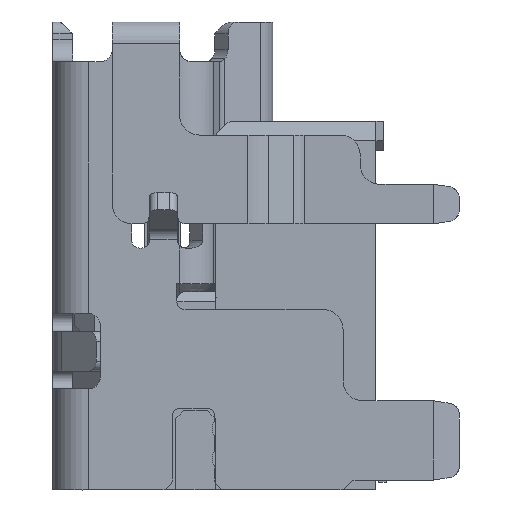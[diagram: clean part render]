
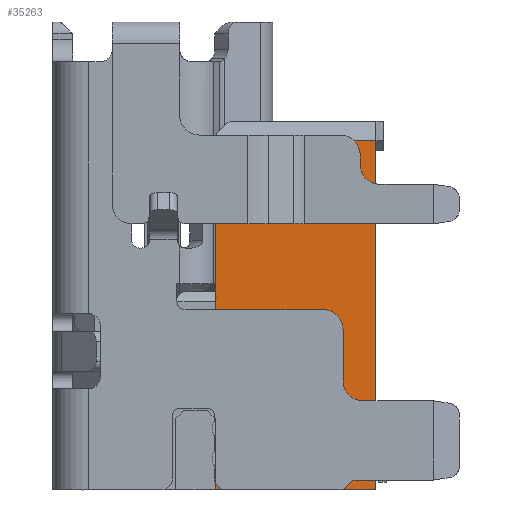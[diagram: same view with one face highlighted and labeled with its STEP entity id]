
A CAD part, left-side view. The second image highlights one B-rep face of the part: STEP entity #35263.
In plain terms, the highlighted planar face has unit normal (-1, 0, 0).
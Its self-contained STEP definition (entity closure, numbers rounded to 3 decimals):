
#2791 = CARTESIAN_POINT ( 'NONE',  ( -6.95, -3.575, -4.9 ) ) ;
#2960 = EDGE_LOOP ( 'NONE', ( #64803, #53405, #57798, #7119, #57390 ) ) ;
#3508 = LINE ( 'NONE', #2791, #50852 ) ;
#7119 = ORIENTED_EDGE ( 'NONE', *, *, #30680, .T. ) ;
#8371 = EDGE_CURVE ( 'NONE', #31630, #37756, #25866, .T. ) ;
#15078 = CARTESIAN_POINT ( 'NONE',  ( -6.95, -7.625, -4.65 ) ) ;
#21367 = DIRECTION ( 'NONE',  ( 0., 0., -1. ) ) ;
#25866 = LINE ( 'NONE', #26198, #50155 ) ;
#26198 = CARTESIAN_POINT ( 'NONE',  ( -6.95, -5.6, -9.3 ) ) ;
#26658 = LINE ( 'NONE', #15078, #41161 ) ;
#30680 = EDGE_CURVE ( 'NONE', #51789, #47878, #3508, .T. ) ;
#31224 = CARTESIAN_POINT ( 'NONE',  ( -6.95, -3.575, -0.5 ) ) ;
#31630 = VERTEX_POINT ( 'NONE', #64844 ) ;
#31987 = DIRECTION ( 'NONE',  ( 0., -1., 0. ) ) ;
#34311 = CARTESIAN_POINT ( 'NONE',  ( -6.95, -3.494, -9.476 ) ) ;
#34691 = DIRECTION ( 'NONE',  ( 0., -1., 0. ) ) ;
#35075 = DIRECTION ( 'NONE',  ( 0., 0., -1. ) ) ;
#35263 = ADVANCED_FACE ( 'NONE', ( #49933 ), #57509, .T. ) ;
#35579 = CARTESIAN_POINT ( 'NONE',  ( -6.95, -3.575, -4.5 ) ) ;
#37756 = VERTEX_POINT ( 'NONE', #63409 ) ;
#39363 = CARTESIAN_POINT ( 'NONE',  ( -6.95, -7.625, -0.5 ) ) ;
#41161 = VECTOR ( 'NONE', #65431, 1000. ) ;
#43654 = EDGE_CURVE ( 'NONE', #47878, #31630, #64897, .T. ) ;
#45292 = EDGE_CURVE ( 'NONE', #52387, #51789, #66682, .T. ) ;
#47878 = VERTEX_POINT ( 'NONE', #35579 ) ;
#49933 = FACE_OUTER_BOUND ( 'NONE', #2960, .T. ) ;
#50155 = VECTOR ( 'NONE', #31987, 1000. ) ;
#50852 = VECTOR ( 'NONE', #35075, 1000. ) ;
#50974 = EDGE_CURVE ( 'NONE', #37756, #52387, #26658, .T. ) ;
#51789 = VERTEX_POINT ( 'NONE', #31224 ) ;
#52387 = VERTEX_POINT ( 'NONE', #39363 ) ;
#53405 = ORIENTED_EDGE ( 'NONE', *, *, #50974, .T. ) ;
#53669 = CARTESIAN_POINT ( 'NONE',  ( -6.95, -3.575, -4.9 ) ) ;
#56450 = DIRECTION ( 'NONE',  ( -1., 0., 0. ) ) ;
#57390 = ORIENTED_EDGE ( 'NONE', *, *, #43654, .T. ) ;
#57509 = PLANE ( 'NONE',  #69052 ) ;
#57798 = ORIENTED_EDGE ( 'NONE', *, *, #45292, .T. ) ;
#59865 = VECTOR ( 'NONE', #62618, 1000. ) ;
#60520 = CARTESIAN_POINT ( 'NONE',  ( -6.95, -5.6, -0.5 ) ) ;
#62618 = DIRECTION ( 'NONE',  ( 0., 1., 0. ) ) ;
#63409 = CARTESIAN_POINT ( 'NONE',  ( -6.95, -7.625, -9.3 ) ) ;
#64534 = VECTOR ( 'NONE', #21367, 1000. ) ;
#64803 = ORIENTED_EDGE ( 'NONE', *, *, #8371, .T. ) ;
#64844 = CARTESIAN_POINT ( 'NONE',  ( -6.95, -3.575, -9.3 ) ) ;
#64897 = LINE ( 'NONE', #53669, #64534 ) ;
#65431 = DIRECTION ( 'NONE',  ( 0., 0., 1. ) ) ;
#66682 = LINE ( 'NONE', #60520, #59865 ) ;
#69052 = AXIS2_PLACEMENT_3D ( 'NONE', #34311, #56450, #34691 ) ;
